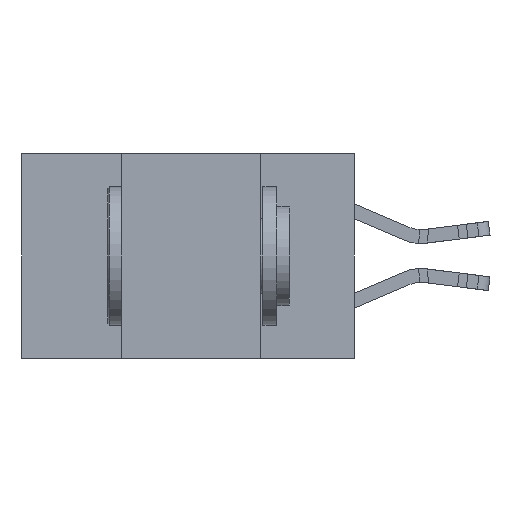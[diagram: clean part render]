
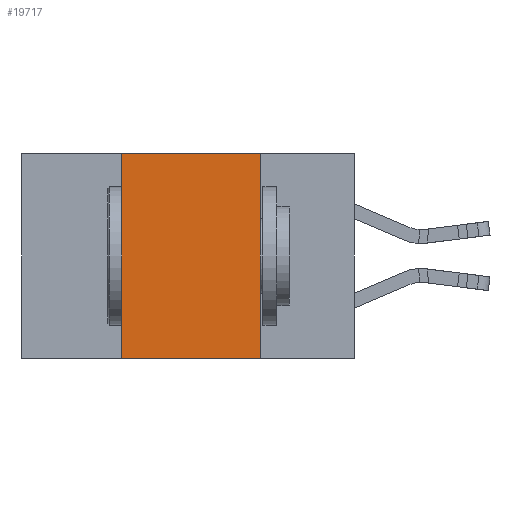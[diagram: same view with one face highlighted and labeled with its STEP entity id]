
A CAD part, left-side view. The second image highlights one B-rep face of the part: STEP entity #19717.
In plain terms, the highlighted planar face has unit normal (-1, 0, 0).
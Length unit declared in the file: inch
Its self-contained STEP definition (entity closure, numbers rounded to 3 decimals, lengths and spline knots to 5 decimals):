
#431 = DIRECTION ( 'NONE',  ( 0., 0., -1. ) ) ;
#890 = ORIENTED_EDGE ( 'NONE', *, *, #11979, .F. ) ;
#2517 = VERTEX_POINT ( 'NONE', #13642 ) ;
#2737 = EDGE_CURVE ( 'NONE', #8878, #6409, #28041, .T. ) ;
#3663 = DIRECTION ( 'NONE',  ( 0., -1., 0. ) ) ;
#4750 = CARTESIAN_POINT ( 'NONE',  ( 0., 0.17, 0. ) ) ;
#6224 = ORIENTED_EDGE ( 'NONE', *, *, #24105, .F. ) ;
#6409 = VERTEX_POINT ( 'NONE', #7219 ) ;
#6815 = VECTOR ( 'NONE', #23067, 39.37008 ) ;
#6845 = VERTEX_POINT ( 'NONE', #22774 ) ;
#7219 = CARTESIAN_POINT ( 'NONE',  ( 0., 0.17, -0.37 ) ) ;
#8878 = VERTEX_POINT ( 'NONE', #25522 ) ;
#10066 = DIRECTION ( 'NONE',  ( 0., 0., -1. ) ) ;
#11979 = EDGE_CURVE ( 'NONE', #8878, #2517, #30058, .T. ) ;
#13636 = CARTESIAN_POINT ( 'NONE',  ( 0., 0.6, 0. ) ) ;
#13642 = CARTESIAN_POINT ( 'NONE',  ( 0., 0.42, 0. ) ) ;
#15714 = VECTOR ( 'NONE', #10066, 39.37008 ) ;
#15816 = ORIENTED_EDGE ( 'NONE', *, *, #2737, .T. ) ;
#16324 = DIRECTION ( 'NONE',  ( 1., 0., 0. ) ) ;
#19334 = FACE_OUTER_BOUND ( 'NONE', #22946, .T. ) ;
#19717 = ADVANCED_FACE ( 'NONE', ( #19334 ), #29565, .F. ) ;
#20546 = LINE ( 'NONE', #22298, #33743 ) ;
#20657 = AXIS2_PLACEMENT_3D ( 'NONE', #13636, #16324, #431 ) ;
#21271 = ORIENTED_EDGE ( 'NONE', *, *, #32718, .F. ) ;
#21631 = CARTESIAN_POINT ( 'NONE',  ( 0., 0.42, 0. ) ) ;
#22014 = LINE ( 'NONE', #4750, #15714 ) ;
#22298 = CARTESIAN_POINT ( 'NONE',  ( 0., 0.6, 0. ) ) ;
#22774 = CARTESIAN_POINT ( 'NONE',  ( 0., 0.17, 0. ) ) ;
#22946 = EDGE_LOOP ( 'NONE', ( #6224, #21271, #890, #15816 ) ) ;
#22954 = CARTESIAN_POINT ( 'NONE',  ( 0., 0.6, -0.37 ) ) ;
#23043 = VECTOR ( 'NONE', #24284, 39.37008 ) ;
#23067 = DIRECTION ( 'NONE',  ( 0., -1., 0. ) ) ;
#24105 = EDGE_CURVE ( 'NONE', #6845, #6409, #22014, .T. ) ;
#24284 = DIRECTION ( 'NONE',  ( 0., 0., 1. ) ) ;
#25522 = CARTESIAN_POINT ( 'NONE',  ( 0., 0.42, -0.37 ) ) ;
#28041 = LINE ( 'NONE', #22954, #6815 ) ;
#29565 = PLANE ( 'NONE',  #20657 ) ;
#30058 = LINE ( 'NONE', #21631, #23043 ) ;
#32718 = EDGE_CURVE ( 'NONE', #2517, #6845, #20546, .T. ) ;
#33743 = VECTOR ( 'NONE', #3663, 39.37008 ) ;
